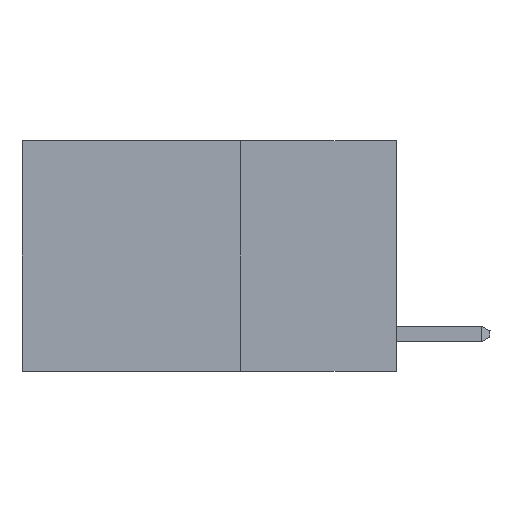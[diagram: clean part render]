
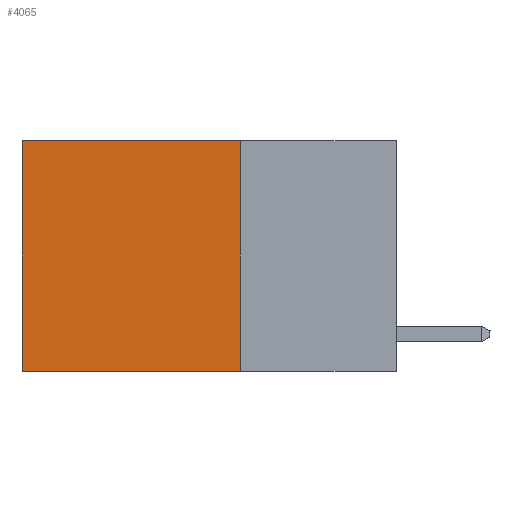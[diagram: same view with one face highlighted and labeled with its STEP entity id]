
A CAD part, left-side view. The second image highlights one B-rep face of the part: STEP entity #4065.
In plain terms, the highlighted planar face has unit normal (-1, 0, 0).
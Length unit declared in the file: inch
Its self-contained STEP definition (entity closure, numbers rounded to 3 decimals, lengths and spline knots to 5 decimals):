
#533 = CARTESIAN_POINT ( 'NONE',  ( 0.2625, 0.6, 0. ) ) ;
#1806 = VECTOR ( 'NONE', #16916, 39.37008 ) ;
#2347 = VECTOR ( 'NONE', #4688, 39.37008 ) ;
#2450 = ORIENTED_EDGE ( 'NONE', *, *, #5302, .F. ) ;
#2513 = EDGE_LOOP ( 'NONE', ( #4099, #2450, #12801, #11614 ) ) ;
#3613 = VERTEX_POINT ( 'NONE', #8644 ) ;
#4065 = ADVANCED_FACE ( 'NONE', ( #13458 ), #4089, .F. ) ;
#4089 = PLANE ( 'NONE',  #16690 ) ;
#4099 = ORIENTED_EDGE ( 'NONE', *, *, #15155, .T. ) ;
#4688 = DIRECTION ( 'NONE',  ( 0., 0., -1. ) ) ;
#5302 = EDGE_CURVE ( 'NONE', #6209, #14067, #9200, .T. ) ;
#5408 = LINE ( 'NONE', #17290, #2347 ) ;
#6209 = VERTEX_POINT ( 'NONE', #9492 ) ;
#6786 = DIRECTION ( 'NONE',  ( 0., 0., -1. ) ) ;
#7242 = EDGE_CURVE ( 'NONE', #3613, #14900, #12181, .T. ) ;
#7783 = CARTESIAN_POINT ( 'NONE',  ( 0.2625, 0.6, -0.37 ) ) ;
#8629 = CARTESIAN_POINT ( 'NONE',  ( 0.2625, 0.6, 0. ) ) ;
#8644 = CARTESIAN_POINT ( 'NONE',  ( 0.2625, 0.25, 0. ) ) ;
#9200 = LINE ( 'NONE', #14321, #1806 ) ;
#9492 = CARTESIAN_POINT ( 'NONE',  ( 0.2625, 0.25, -0.37 ) ) ;
#9992 = VECTOR ( 'NONE', #15365, 39.37008 ) ;
#11095 = CARTESIAN_POINT ( 'NONE',  ( 0.2625, 0.25, 0. ) ) ;
#11511 = DIRECTION ( 'NONE',  ( 0., 0., -1. ) ) ;
#11614 = ORIENTED_EDGE ( 'NONE', *, *, #7242, .T. ) ;
#12181 = LINE ( 'NONE', #15182, #9992 ) ;
#12801 = ORIENTED_EDGE ( 'NONE', *, *, #16805, .F. ) ;
#13458 = FACE_OUTER_BOUND ( 'NONE', #2513, .T. ) ;
#14067 = VERTEX_POINT ( 'NONE', #7783 ) ;
#14321 = CARTESIAN_POINT ( 'NONE',  ( 0.2625, 0.25, -0.37 ) ) ;
#14900 = VERTEX_POINT ( 'NONE', #8629 ) ;
#15136 = DIRECTION ( 'NONE',  ( 1., 0., 0. ) ) ;
#15155 = EDGE_CURVE ( 'NONE', #14900, #14067, #15472, .T. ) ;
#15182 = CARTESIAN_POINT ( 'NONE',  ( 0.2625, 0.25, 0. ) ) ;
#15365 = DIRECTION ( 'NONE',  ( 0., 1., 0. ) ) ;
#15472 = LINE ( 'NONE', #533, #16352 ) ;
#16352 = VECTOR ( 'NONE', #11511, 39.37008 ) ;
#16690 = AXIS2_PLACEMENT_3D ( 'NONE', #11095, #15136, #6786 ) ;
#16805 = EDGE_CURVE ( 'NONE', #3613, #6209, #5408, .T. ) ;
#16916 = DIRECTION ( 'NONE',  ( 0., 1., 0. ) ) ;
#17290 = CARTESIAN_POINT ( 'NONE',  ( 0.2625, 0.25, 0. ) ) ;
